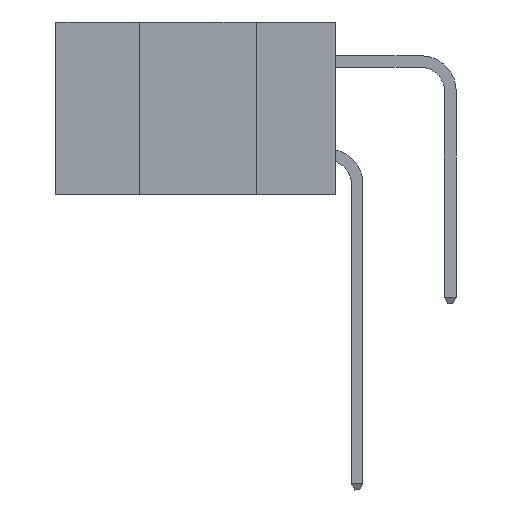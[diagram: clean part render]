
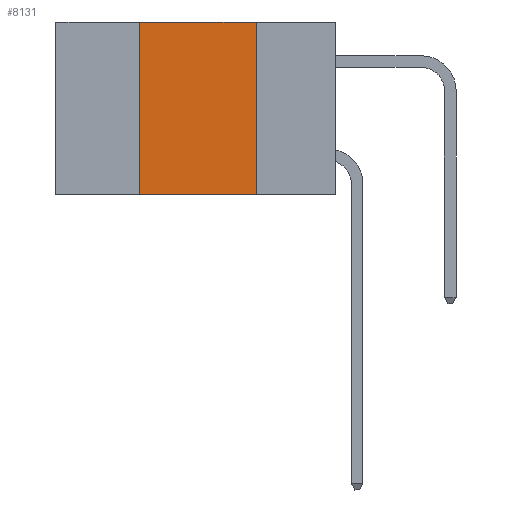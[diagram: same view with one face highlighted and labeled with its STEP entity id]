
A CAD part, left-side view. The second image highlights one B-rep face of the part: STEP entity #8131.
In plain terms, the highlighted planar face has unit normal (-1, 0, 0).
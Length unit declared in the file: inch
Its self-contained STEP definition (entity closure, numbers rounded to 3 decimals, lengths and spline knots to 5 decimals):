
#632 = VECTOR ( 'NONE', #10088, 39.37008 ) ;
#1883 = LINE ( 'NONE', #12519, #19778 ) ;
#3972 = EDGE_CURVE ( 'NONE', #14766, #20809, #13116, .T. ) ;
#5304 = CARTESIAN_POINT ( 'NONE',  ( 0., 0.6, 0. ) ) ;
#5400 = ORIENTED_EDGE ( 'NONE', *, *, #7649, .F. ) ;
#5745 = LINE ( 'NONE', #16889, #9351 ) ;
#5925 = DIRECTION ( 'NONE',  ( 0., 0., -1. ) ) ;
#6294 = CARTESIAN_POINT ( 'NONE',  ( 0., 0.6, 0. ) ) ;
#6852 = DIRECTION ( 'NONE',  ( 0., 0., 1. ) ) ;
#7059 = EDGE_CURVE ( 'NONE', #17446, #20880, #22793, .T. ) ;
#7064 = AXIS2_PLACEMENT_3D ( 'NONE', #5304, #17736, #17956 ) ;
#7649 = EDGE_CURVE ( 'NONE', #14766, #17446, #1883, .T. ) ;
#8131 = ADVANCED_FACE ( 'NONE', ( #14181 ), #16199, .F. ) ;
#8413 = ORIENTED_EDGE ( 'NONE', *, *, #9524, .F. ) ;
#9351 = VECTOR ( 'NONE', #5925, 39.37008 ) ;
#9524 = EDGE_CURVE ( 'NONE', #20880, #20809, #5745, .T. ) ;
#9751 = VECTOR ( 'NONE', #19067, 39.37008 ) ;
#10088 = DIRECTION ( 'NONE',  ( 0., -1., 0. ) ) ;
#10894 = CARTESIAN_POINT ( 'NONE',  ( 0., 0.17, 0. ) ) ;
#12163 = CARTESIAN_POINT ( 'NONE',  ( 0., 0.42, 0. ) ) ;
#12191 = EDGE_LOOP ( 'NONE', ( #8413, #14724, #5400, #16628 ) ) ;
#12519 = CARTESIAN_POINT ( 'NONE',  ( 0., 0.42, 0. ) ) ;
#13116 = LINE ( 'NONE', #17424, #9751 ) ;
#14181 = FACE_OUTER_BOUND ( 'NONE', #12191, .T. ) ;
#14724 = ORIENTED_EDGE ( 'NONE', *, *, #7059, .F. ) ;
#14766 = VERTEX_POINT ( 'NONE', #15774 ) ;
#15774 = CARTESIAN_POINT ( 'NONE',  ( 0., 0.42, -0.37 ) ) ;
#16054 = CARTESIAN_POINT ( 'NONE',  ( 0., 0.17, -0.37 ) ) ;
#16199 = PLANE ( 'NONE',  #7064 ) ;
#16628 = ORIENTED_EDGE ( 'NONE', *, *, #3972, .T. ) ;
#16889 = CARTESIAN_POINT ( 'NONE',  ( 0., 0.17, 0. ) ) ;
#17424 = CARTESIAN_POINT ( 'NONE',  ( 0., 0.6, -0.37 ) ) ;
#17446 = VERTEX_POINT ( 'NONE', #12163 ) ;
#17736 = DIRECTION ( 'NONE',  ( 1., 0., 0. ) ) ;
#17956 = DIRECTION ( 'NONE',  ( 0., 0., -1. ) ) ;
#19067 = DIRECTION ( 'NONE',  ( 0., -1., 0. ) ) ;
#19778 = VECTOR ( 'NONE', #6852, 39.37008 ) ;
#20809 = VERTEX_POINT ( 'NONE', #16054 ) ;
#20880 = VERTEX_POINT ( 'NONE', #10894 ) ;
#22793 = LINE ( 'NONE', #6294, #632 ) ;
